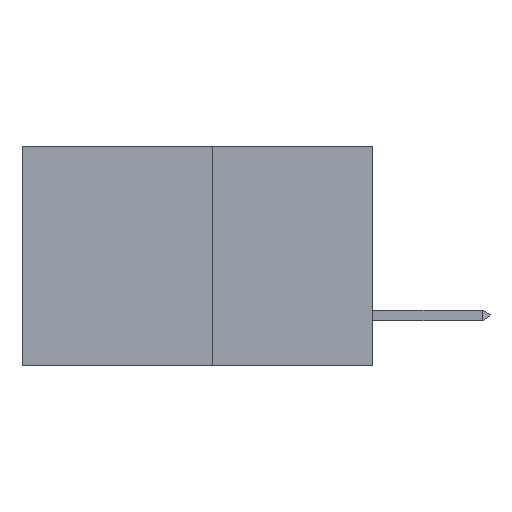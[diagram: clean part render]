
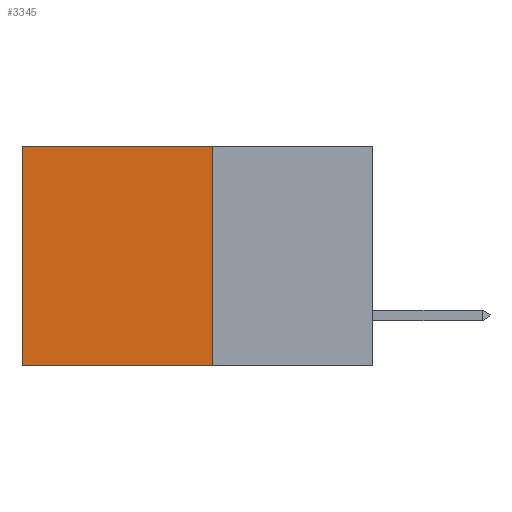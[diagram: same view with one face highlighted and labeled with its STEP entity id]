
A CAD part, left-side view. The second image highlights one B-rep face of the part: STEP entity #3345.
In plain terms, the highlighted planar face has unit normal (-1, 0, 0).
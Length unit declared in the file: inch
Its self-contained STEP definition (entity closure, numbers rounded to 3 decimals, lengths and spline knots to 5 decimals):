
#210 = AXIS2_PLACEMENT_3D ( 'NONE', #6682, #10684, #4873 ) ;
#331 = ORIENTED_EDGE ( 'NONE', *, *, #6187, .F. ) ;
#460 = ORIENTED_EDGE ( 'NONE', *, *, #2921, .F. ) ;
#624 = VECTOR ( 'NONE', #1780, 39.37008 ) ;
#805 = CARTESIAN_POINT ( 'NONE',  ( 0.277, 0.59, -0.37 ) ) ;
#949 = LINE ( 'NONE', #10126, #6229 ) ;
#1659 = VERTEX_POINT ( 'NONE', #6059 ) ;
#1780 = DIRECTION ( 'NONE',  ( 0., 0., -1. ) ) ;
#2009 = CARTESIAN_POINT ( 'NONE',  ( 0.277, 0.27, -0.37 ) ) ;
#2745 = VERTEX_POINT ( 'NONE', #11744 ) ;
#2921 = EDGE_CURVE ( 'NONE', #7239, #11666, #10124, .T. ) ;
#3145 = DIRECTION ( 'NONE',  ( 0., 1., 0. ) ) ;
#3345 = ADVANCED_FACE ( 'NONE', ( #7816 ), #8708, .F. ) ;
#3492 = EDGE_CURVE ( 'NONE', #1659, #2745, #949, .T. ) ;
#3511 = CARTESIAN_POINT ( 'NONE',  ( 0.277, 0.27, -0.37 ) ) ;
#3922 = EDGE_CURVE ( 'NONE', #2745, #11666, #5902, .T. ) ;
#4486 = DIRECTION ( 'NONE',  ( 0., 0., -1. ) ) ;
#4553 = EDGE_LOOP ( 'NONE', ( #6799, #460, #331, #7464 ) ) ;
#4873 = DIRECTION ( 'NONE',  ( 0., 0., -1. ) ) ;
#5010 = DIRECTION ( 'NONE',  ( 0., 1., 0. ) ) ;
#5902 = LINE ( 'NONE', #805, #624 ) ;
#5992 = VECTOR ( 'NONE', #4486, 39.37008 ) ;
#6059 = CARTESIAN_POINT ( 'NONE',  ( 0.277, 0.27, 0. ) ) ;
#6187 = EDGE_CURVE ( 'NONE', #1659, #7239, #8982, .T. ) ;
#6229 = VECTOR ( 'NONE', #3145, 39.37008 ) ;
#6682 = CARTESIAN_POINT ( 'NONE',  ( 0.277, 0.27, -0.37 ) ) ;
#6799 = ORIENTED_EDGE ( 'NONE', *, *, #3922, .T. ) ;
#6946 = CARTESIAN_POINT ( 'NONE',  ( 0.277, 0.27, -0.37 ) ) ;
#7239 = VERTEX_POINT ( 'NONE', #6946 ) ;
#7464 = ORIENTED_EDGE ( 'NONE', *, *, #3492, .T. ) ;
#7816 = FACE_OUTER_BOUND ( 'NONE', #4553, .T. ) ;
#8708 = PLANE ( 'NONE',  #210 ) ;
#8982 = LINE ( 'NONE', #3511, #5992 ) ;
#10124 = LINE ( 'NONE', #2009, #12440 ) ;
#10126 = CARTESIAN_POINT ( 'NONE',  ( 0.277, 0.27, 0. ) ) ;
#10684 = DIRECTION ( 'NONE',  ( 1., 0., 0. ) ) ;
#10863 = CARTESIAN_POINT ( 'NONE',  ( 0.277, 0.59, -0.37 ) ) ;
#11666 = VERTEX_POINT ( 'NONE', #10863 ) ;
#11744 = CARTESIAN_POINT ( 'NONE',  ( 0.277, 0.59, 0. ) ) ;
#12440 = VECTOR ( 'NONE', #5010, 39.37008 ) ;
